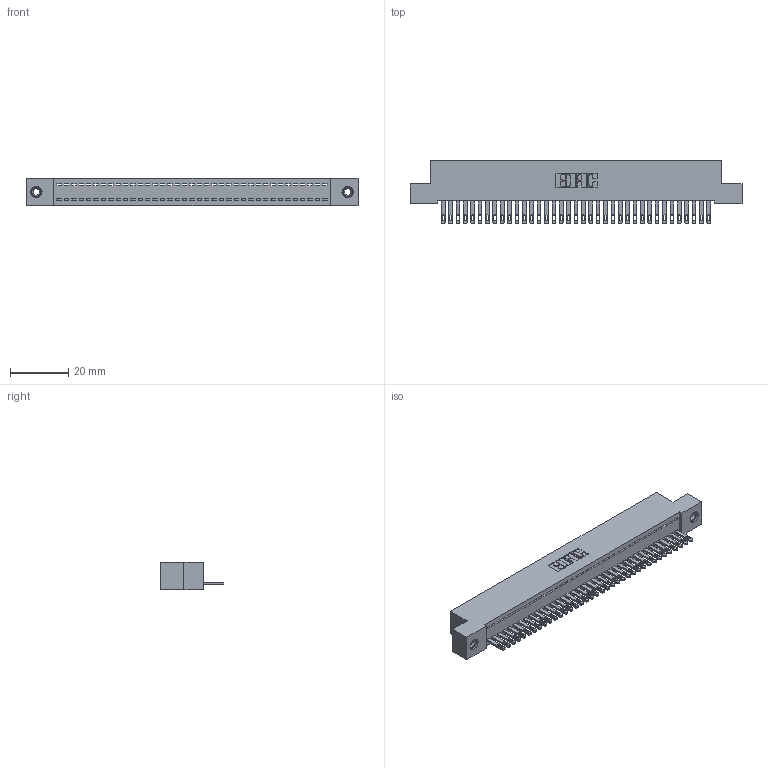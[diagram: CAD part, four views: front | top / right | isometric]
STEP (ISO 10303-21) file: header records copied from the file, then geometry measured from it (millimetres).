
FILE_DESCRIPTION (( 'STEP AP203' ), '1' );
FILE_NAME ('892-037-500-108.STEP', '2020-09-21T16:03:44', ( '' ), ( '' ), 'SwSTEP 2.0', 'SolidWorks 2020', '' );
FILE_SCHEMA (( 'CONFIG_CONTROL_DESIGN' ));
Length unit declared in the file: inch
Products named in the file (4): 345-292-001_345-293-100; 842 Part_TI; 892-037-500-108; 345-250-001_345-250-003-102
Assembly tree (40 placements, depth 2):
  892-037-500-108
    842 Part_TI
    345-292-001_345-293-100  x37
    345-250-001_345-250-003-102  x2
Bounding box: 114.3 x 21.85 x 9.4 mm (x, y, z)
Volume: 10020.6 mm3; surface area: 14712.1 mm2
Topology: 40 solids, 40 shells, 2168 faces, 6651 edges, 4426 vertices
Faces by surface type: plane 1430, cylinder 722, cone 12, torus 4
Entity records: 24250 total; most frequent: CARTESIAN_POINT 4164, ORIENTED_EDGE 4130, DIRECTION 3557, EDGE_CURVE 2065, LINE 1913, VECTOR 1913, VERTEX_POINT 1372, AXIS2_PLACEMENT_3D 822
